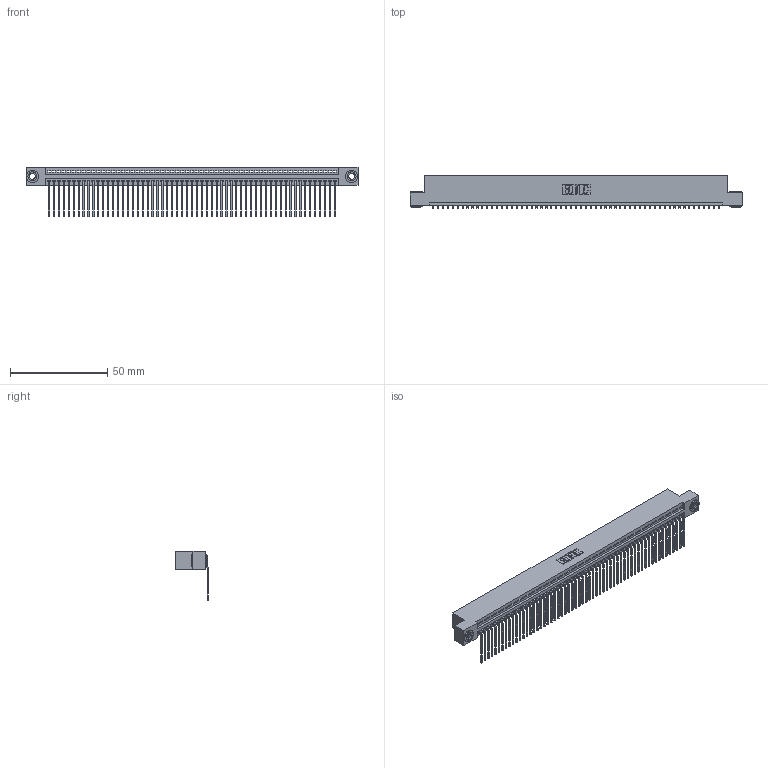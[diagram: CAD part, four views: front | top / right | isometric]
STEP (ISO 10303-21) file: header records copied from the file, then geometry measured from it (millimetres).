
FILE_DESCRIPTION (( 'STEP AP203' ), '1' );
FILE_NAME ('345-059-559-103.STEP', '2019-10-10T20:57:42', ( '' ), ( '' ), 'SwSTEP 2.0', 'SolidWorks 2016', '' );
FILE_SCHEMA (( 'CONFIG_CONTROL_DESIGN' ));
Length unit declared in the file: inch
Products named in the file (4): 345-250-002_345-250-002-102; 345 Part_Flush Mounting Lugs - 0.156 Dia-TH; 345-059-559-103; 345-292-001_558 559 Tail - 1
Assembly tree (62 placements, depth 2):
  345-059-559-103
    345 Part_Flush Mounting Lugs - 0.156 Dia-TH
    345-292-001_558 559 Tail - 1  x59
    345-250-002_345-250-002-102  x2
Bounding box: 171.07 x 16.75 x 25.53 mm (x, y, z)
Volume: 16603.5 mm3; surface area: 23665.2 mm2
Topology: 62 solids, 62 shells, 3704 faces, 11155 edges, 7354 vertices
Faces by surface type: plane 2568, cylinder 1128, cone 8
Entity records: 42850 total; most frequent: CARTESIAN_POINT 7400, ORIENTED_EDGE 7386, DIRECTION 6469, EDGE_CURVE 3693, VECTOR 3301, LINE 3301, VERTEX_POINT 2458, AXIS2_PLACEMENT_3D 1584
